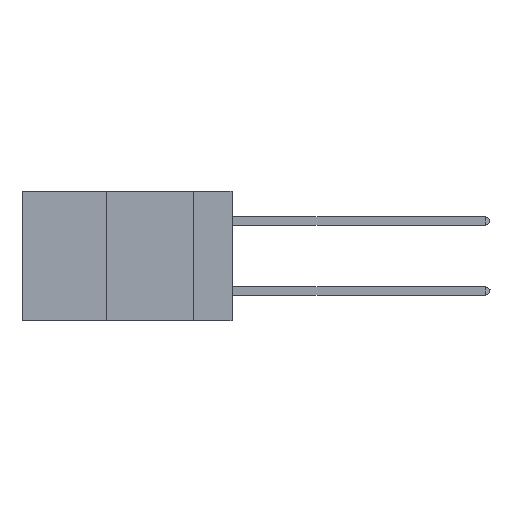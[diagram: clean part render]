
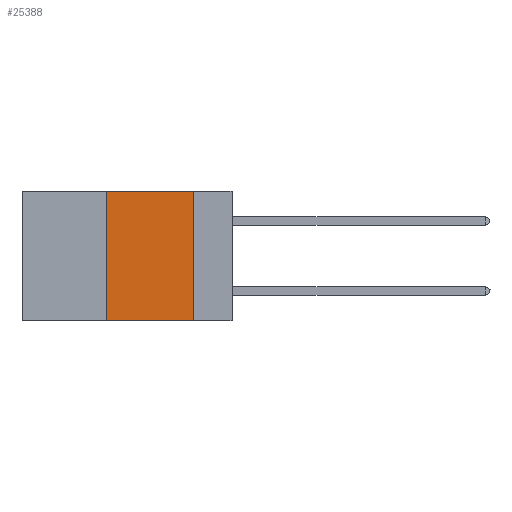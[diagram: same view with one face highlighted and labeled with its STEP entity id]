
A CAD part, left-side view. The second image highlights one B-rep face of the part: STEP entity #25388.
In plain terms, the highlighted planar face has unit normal (-1, 0, 0).
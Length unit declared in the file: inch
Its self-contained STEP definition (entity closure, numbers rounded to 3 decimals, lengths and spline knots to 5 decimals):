
#289 = DIRECTION ( 'NONE',  ( 0., 0., -1. ) ) ;
#300 = CARTESIAN_POINT ( 'NONE',  ( 0., 0.11, 0. ) ) ;
#1346 = ORIENTED_EDGE ( 'NONE', *, *, #26061, .F. ) ;
#2085 = DIRECTION ( 'NONE',  ( 0., 0., -1. ) ) ;
#3042 = AXIS2_PLACEMENT_3D ( 'NONE', #22843, #9057, #289 ) ;
#4333 = VERTEX_POINT ( 'NONE', #34447 ) ;
#7683 = CARTESIAN_POINT ( 'NONE',  ( 0., 0.36, -0.37 ) ) ;
#9057 = DIRECTION ( 'NONE',  ( 1., 0., 0. ) ) ;
#9753 = LINE ( 'NONE', #26492, #30594 ) ;
#11308 = CARTESIAN_POINT ( 'NONE',  ( 0., 0.6, 0. ) ) ;
#11486 = PLANE ( 'NONE',  #3042 ) ;
#13928 = ORIENTED_EDGE ( 'NONE', *, *, #15661, .F. ) ;
#14898 = VECTOR ( 'NONE', #2085, 39.37008 ) ;
#15194 = LINE ( 'NONE', #24297, #19301 ) ;
#15661 = EDGE_CURVE ( 'NONE', #24191, #4333, #15194, .T. ) ;
#17437 = FACE_OUTER_BOUND ( 'NONE', #28894, .T. ) ;
#18482 = VERTEX_POINT ( 'NONE', #300 ) ;
#18507 = LINE ( 'NONE', #29851, #14898 ) ;
#19301 = VECTOR ( 'NONE', #32117, 39.37008 ) ;
#20414 = VERTEX_POINT ( 'NONE', #28327 ) ;
#21107 = DIRECTION ( 'NONE',  ( 0., -1., 0. ) ) ;
#22119 = LINE ( 'NONE', #11308, #31034 ) ;
#22843 = CARTESIAN_POINT ( 'NONE',  ( 0., 0.6, 0. ) ) ;
#24182 = EDGE_CURVE ( 'NONE', #18482, #20414, #18507, .T. ) ;
#24191 = VERTEX_POINT ( 'NONE', #7683 ) ;
#24297 = CARTESIAN_POINT ( 'NONE',  ( 0., 0.36, 0. ) ) ;
#25388 = ADVANCED_FACE ( 'NONE', ( #17437 ), #11486, .F. ) ;
#26061 = EDGE_CURVE ( 'NONE', #4333, #18482, #22119, .T. ) ;
#26492 = CARTESIAN_POINT ( 'NONE',  ( 0., 0.6, -0.37 ) ) ;
#28068 = DIRECTION ( 'NONE',  ( 0., -1., 0. ) ) ;
#28327 = CARTESIAN_POINT ( 'NONE',  ( 0., 0.11, -0.37 ) ) ;
#28620 = ORIENTED_EDGE ( 'NONE', *, *, #30946, .T. ) ;
#28894 = EDGE_LOOP ( 'NONE', ( #34695, #1346, #13928, #28620 ) ) ;
#29851 = CARTESIAN_POINT ( 'NONE',  ( 0., 0.11, 0. ) ) ;
#30594 = VECTOR ( 'NONE', #21107, 39.37008 ) ;
#30946 = EDGE_CURVE ( 'NONE', #24191, #20414, #9753, .T. ) ;
#31034 = VECTOR ( 'NONE', #28068, 39.37008 ) ;
#32117 = DIRECTION ( 'NONE',  ( 0., 0., 1. ) ) ;
#34447 = CARTESIAN_POINT ( 'NONE',  ( 0., 0.36, 0. ) ) ;
#34695 = ORIENTED_EDGE ( 'NONE', *, *, #24182, .F. ) ;
